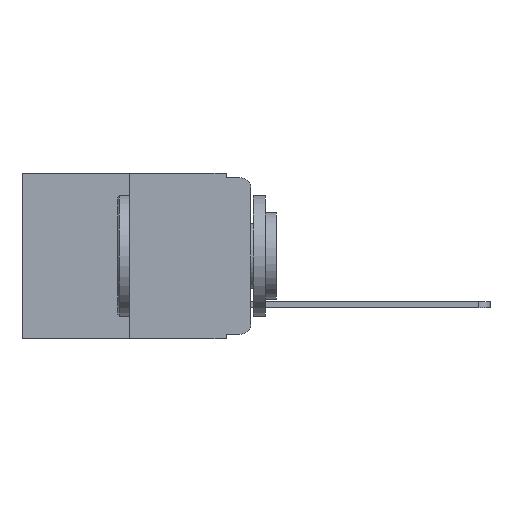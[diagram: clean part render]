
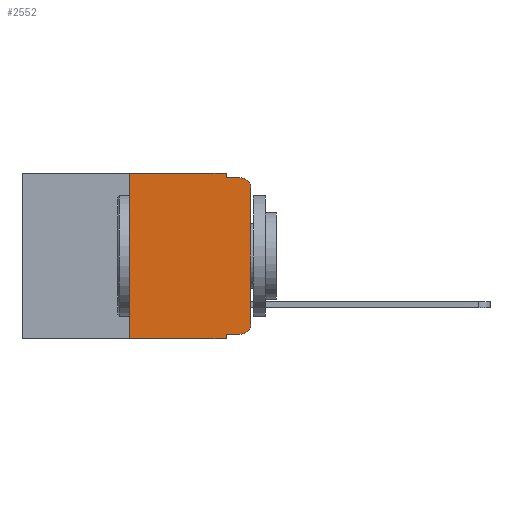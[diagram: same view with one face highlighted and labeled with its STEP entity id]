
A CAD part, left-side view. The second image highlights one B-rep face of the part: STEP entity #2552.
In plain terms, the highlighted planar face has unit normal (-1, 0, 0).
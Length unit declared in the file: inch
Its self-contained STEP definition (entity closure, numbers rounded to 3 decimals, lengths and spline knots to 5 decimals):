
#238 = CARTESIAN_POINT ( 'NONE',  ( 0., 0., -0.03 ) ) ;
#256 = AXIS2_PLACEMENT_3D ( 'NONE', #12124, #2257, #13582 ) ;
#445 = VERTEX_POINT ( 'NONE', #6322 ) ;
#596 = VERTEX_POINT ( 'NONE', #238 ) ;
#796 = VECTOR ( 'NONE', #14124, 39.37008 ) ;
#1048 = VERTEX_POINT ( 'NONE', #15451 ) ;
#1116 = CARTESIAN_POINT ( 'NONE',  ( 0., 0.473, 0. ) ) ;
#1142 = CARTESIAN_POINT ( 'NONE',  ( 0., 0.051, -0.333 ) ) ;
#1143 = EDGE_CURVE ( 'NONE', #15511, #12961, #7465, .T. ) ;
#1232 = VECTOR ( 'NONE', #3169, 39.37008 ) ;
#1883 = VERTEX_POINT ( 'NONE', #9413 ) ;
#1954 = EDGE_CURVE ( 'NONE', #13876, #445, #6091, .T. ) ;
#2257 = DIRECTION ( 'NONE',  ( -1., 0., 0. ) ) ;
#2287 = VECTOR ( 'NONE', #6758, 39.37008 ) ;
#2517 = ORIENTED_EDGE ( 'NONE', *, *, #3141, .F. ) ;
#2552 = ADVANCED_FACE ( 'NONE', ( #19248 ), #11236, .F. ) ;
#2914 = DIRECTION ( 'NONE',  ( 0., 0., -1. ) ) ;
#3141 = EDGE_CURVE ( 'NONE', #445, #5375, #13687, .T. ) ;
#3169 = DIRECTION ( 'NONE',  ( 0., -1., 0. ) ) ;
#3687 = VECTOR ( 'NONE', #8855, 39.37008 ) ;
#4122 = DIRECTION ( 'NONE',  ( 0., 0., -1. ) ) ;
#4469 = VERTEX_POINT ( 'NONE', #17986 ) ;
#4727 = CARTESIAN_POINT ( 'NONE',  ( 0., 0., 0. ) ) ;
#4760 = EDGE_CURVE ( 'NONE', #596, #5375, #15630, .T. ) ;
#4887 = VECTOR ( 'NONE', #2914, 39.37008 ) ;
#5030 = ORIENTED_EDGE ( 'NONE', *, *, #17203, .T. ) ;
#5375 = VERTEX_POINT ( 'NONE', #14385 ) ;
#5800 = AXIS2_PLACEMENT_3D ( 'NONE', #12043, #13633, #4122 ) ;
#5900 = CARTESIAN_POINT ( 'NONE',  ( 0., 0.25, -0.343 ) ) ;
#6091 = LINE ( 'NONE', #19787, #8905 ) ;
#6322 = CARTESIAN_POINT ( 'NONE',  ( 0., 0.051, -0.01 ) ) ;
#6758 = DIRECTION ( 'NONE',  ( 0., 0., 1. ) ) ;
#6899 = CARTESIAN_POINT ( 'NONE',  ( 0., 0.02, -0.333 ) ) ;
#7260 = CARTESIAN_POINT ( 'NONE',  ( 0., 0.473, 0. ) ) ;
#7465 = LINE ( 'NONE', #1142, #10635 ) ;
#7708 = LINE ( 'NONE', #8399, #2287 ) ;
#8180 = CARTESIAN_POINT ( 'NONE',  ( 0., 0.473, -0.343 ) ) ;
#8399 = CARTESIAN_POINT ( 'NONE',  ( 0., 0.25, 0. ) ) ;
#8456 = ORIENTED_EDGE ( 'NONE', *, *, #14112, .F. ) ;
#8855 = DIRECTION ( 'NONE',  ( 0., -1., 0. ) ) ;
#8905 = VECTOR ( 'NONE', #19765, 39.37008 ) ;
#8936 = DIRECTION ( 'NONE',  ( 0., 0., -1. ) ) ;
#9160 = ORIENTED_EDGE ( 'NONE', *, *, #13092, .F. ) ;
#9275 = LINE ( 'NONE', #9604, #4887 ) ;
#9405 = CIRCLE ( 'NONE', #256, 0.02 ) ;
#9413 = CARTESIAN_POINT ( 'NONE',  ( 0., 0., -0.313 ) ) ;
#9509 = VERTEX_POINT ( 'NONE', #5900 ) ;
#9604 = CARTESIAN_POINT ( 'NONE',  ( 0., 0.051, 0. ) ) ;
#9964 = DIRECTION ( 'NONE',  ( 1., 0., 0. ) ) ;
#10103 = LINE ( 'NONE', #8180, #13151 ) ;
#10635 = VECTOR ( 'NONE', #14460, 39.37008 ) ;
#11236 = PLANE ( 'NONE',  #11865 ) ;
#11865 = AXIS2_PLACEMENT_3D ( 'NONE', #1116, #9964, #8936 ) ;
#12043 = CARTESIAN_POINT ( 'NONE',  ( 0., 0.02, -0.03 ) ) ;
#12124 = CARTESIAN_POINT ( 'NONE',  ( 0., 0.02, -0.313 ) ) ;
#12272 = ORIENTED_EDGE ( 'NONE', *, *, #1954, .F. ) ;
#12512 = ORIENTED_EDGE ( 'NONE', *, *, #1143, .T. ) ;
#12909 = EDGE_CURVE ( 'NONE', #9509, #1048, #7708, .T. ) ;
#12961 = VERTEX_POINT ( 'NONE', #6899 ) ;
#13092 = EDGE_CURVE ( 'NONE', #1048, #13876, #19421, .T. ) ;
#13151 = VECTOR ( 'NONE', #15647, 39.37008 ) ;
#13582 = DIRECTION ( 'NONE',  ( 0., 0., -1. ) ) ;
#13633 = DIRECTION ( 'NONE',  ( -1., 0., 0. ) ) ;
#13687 = LINE ( 'NONE', #14300, #1232 ) ;
#13796 = LINE ( 'NONE', #4727, #796 ) ;
#13876 = VERTEX_POINT ( 'NONE', #16490 ) ;
#14081 = ORIENTED_EDGE ( 'NONE', *, *, #12909, .F. ) ;
#14112 = EDGE_CURVE ( 'NONE', #15511, #4469, #9275, .T. ) ;
#14124 = DIRECTION ( 'NONE',  ( 0., 0., 1. ) ) ;
#14300 = CARTESIAN_POINT ( 'NONE',  ( 0., 0.051, -0.01 ) ) ;
#14385 = CARTESIAN_POINT ( 'NONE',  ( 0., 0.02, -0.01 ) ) ;
#14460 = DIRECTION ( 'NONE',  ( 0., -1., 0. ) ) ;
#15451 = CARTESIAN_POINT ( 'NONE',  ( 0., 0.25, 0. ) ) ;
#15511 = VERTEX_POINT ( 'NONE', #18341 ) ;
#15630 = CIRCLE ( 'NONE', #5800, 0.02 ) ;
#15647 = DIRECTION ( 'NONE',  ( 0., -1., 0. ) ) ;
#15856 = ORIENTED_EDGE ( 'NONE', *, *, #19331, .T. ) ;
#16490 = CARTESIAN_POINT ( 'NONE',  ( 0., 0.051, 0. ) ) ;
#17203 = EDGE_CURVE ( 'NONE', #12961, #1883, #9405, .T. ) ;
#17458 = EDGE_LOOP ( 'NONE', ( #15856, #17620, #2517, #12272, #9160, #14081, #19189, #8456, #12512, #5030 ) ) ;
#17620 = ORIENTED_EDGE ( 'NONE', *, *, #4760, .T. ) ;
#17986 = CARTESIAN_POINT ( 'NONE',  ( 0., 0.051, -0.343 ) ) ;
#18341 = CARTESIAN_POINT ( 'NONE',  ( 0., 0.051, -0.333 ) ) ;
#18737 = EDGE_CURVE ( 'NONE', #9509, #4469, #10103, .T. ) ;
#19189 = ORIENTED_EDGE ( 'NONE', *, *, #18737, .T. ) ;
#19248 = FACE_OUTER_BOUND ( 'NONE', #17458, .T. ) ;
#19331 = EDGE_CURVE ( 'NONE', #1883, #596, #13796, .T. ) ;
#19421 = LINE ( 'NONE', #7260, #3687 ) ;
#19765 = DIRECTION ( 'NONE',  ( 0., 0., -1. ) ) ;
#19787 = CARTESIAN_POINT ( 'NONE',  ( 0., 0.051, 0. ) ) ;
